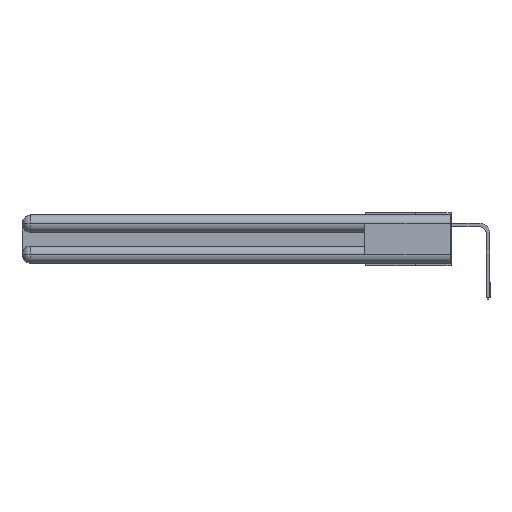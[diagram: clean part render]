
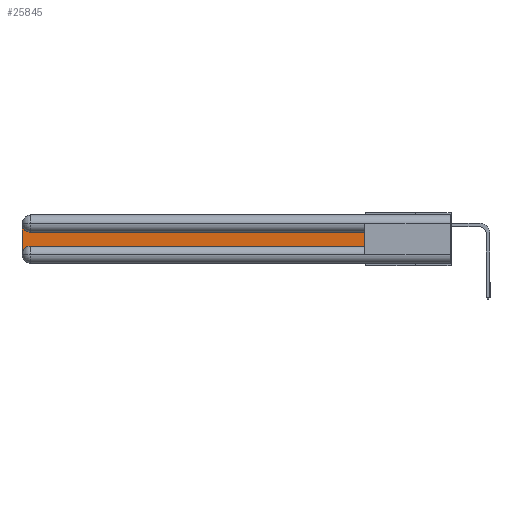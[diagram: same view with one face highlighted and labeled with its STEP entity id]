
A CAD part, left-side view. The second image highlights one B-rep face of the part: STEP entity #25845.
In plain terms, the highlighted planar face has unit normal (-1, 0, 0).
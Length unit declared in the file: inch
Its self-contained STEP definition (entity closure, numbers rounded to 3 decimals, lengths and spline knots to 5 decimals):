
#1119 = ORIENTED_EDGE ( 'NONE', *, *, #12127, .T. ) ;
#1807 = CARTESIAN_POINT ( 'NONE',  ( 0.075, 0.6, -0.1225 ) ) ;
#2072 = DIRECTION ( 'NONE',  ( 1., 0., 0. ) ) ;
#2469 = ORIENTED_EDGE ( 'NONE', *, *, #16069, .T. ) ;
#2662 = DIRECTION ( 'NONE',  ( 0., 0., 1. ) ) ;
#2831 = DIRECTION ( 'NONE',  ( 0., 1., 0. ) ) ;
#3142 = ORIENTED_EDGE ( 'NONE', *, *, #17017, .T. ) ;
#3325 = LINE ( 'NONE', #16458, #4412 ) ;
#3398 = VECTOR ( 'NONE', #2662, 39.37008 ) ;
#3775 = LINE ( 'NONE', #17286, #15225 ) ;
#3799 = EDGE_CURVE ( 'NONE', #9371, #26437, #3325, .T. ) ;
#4103 = VERTEX_POINT ( 'NONE', #1807 ) ;
#4412 = VECTOR ( 'NONE', #5385, 39.37008 ) ;
#5385 = DIRECTION ( 'NONE',  ( 0., -1., 0. ) ) ;
#5454 = AXIS2_PLACEMENT_3D ( 'NONE', #15026, #21813, #8323 ) ;
#5946 = FACE_OUTER_BOUND ( 'NONE', #22293, .T. ) ;
#6740 = CIRCLE ( 'NONE', #21140, 0.06 ) ;
#6820 = CARTESIAN_POINT ( 'NONE',  ( 0.075, 3., -0.1225 ) ) ;
#7042 = CARTESIAN_POINT ( 'NONE',  ( 0.075, 2.94, -0.2175 ) ) ;
#8323 = DIRECTION ( 'NONE',  ( 0., 0., -1. ) ) ;
#9371 = VERTEX_POINT ( 'NONE', #7042 ) ;
#10769 = VERTEX_POINT ( 'NONE', #17745 ) ;
#12127 = EDGE_CURVE ( 'NONE', #26437, #4103, #21660, .T. ) ;
#12393 = CIRCLE ( 'NONE', #5454, 0.06 ) ;
#13222 = EDGE_CURVE ( 'NONE', #4103, #14517, #17979, .T. ) ;
#13375 = CARTESIAN_POINT ( 'NONE',  ( 0.075, 0.6, -0.2175 ) ) ;
#14067 = VECTOR ( 'NONE', #2831, 39.37008 ) ;
#14517 = VERTEX_POINT ( 'NONE', #19823 ) ;
#15016 = ORIENTED_EDGE ( 'NONE', *, *, #17558, .T. ) ;
#15026 = CARTESIAN_POINT ( 'NONE',  ( 0.075, 2.94, -0.0625 ) ) ;
#15225 = VECTOR ( 'NONE', #28755, 39.37008 ) ;
#15980 = PLANE ( 'NONE',  #26422 ) ;
#16069 = EDGE_CURVE ( 'NONE', #10769, #9371, #6740, .T. ) ;
#16458 = CARTESIAN_POINT ( 'NONE',  ( 0.075, 0.6, -0.2175 ) ) ;
#17017 = EDGE_CURVE ( 'NONE', #25446, #10769, #3775, .T. ) ;
#17286 = CARTESIAN_POINT ( 'NONE',  ( 0.075, 3., -0.2175 ) ) ;
#17558 = EDGE_CURVE ( 'NONE', #14517, #25446, #12393, .T. ) ;
#17745 = CARTESIAN_POINT ( 'NONE',  ( 0.075, 3., -0.2775 ) ) ;
#17979 = LINE ( 'NONE', #29601, #14067 ) ;
#18504 = ORIENTED_EDGE ( 'NONE', *, *, #3799, .T. ) ;
#19823 = CARTESIAN_POINT ( 'NONE',  ( 0.075, 2.94, -0.1225 ) ) ;
#21140 = AXIS2_PLACEMENT_3D ( 'NONE', #23126, #23403, #25714 ) ;
#21191 = CARTESIAN_POINT ( 'NONE',  ( 0.075, 0.6, -0.2175 ) ) ;
#21319 = CARTESIAN_POINT ( 'NONE',  ( 0.075, 3., -0.0625 ) ) ;
#21660 = LINE ( 'NONE', #21191, #3398 ) ;
#21813 = DIRECTION ( 'NONE',  ( 1., 0., 0. ) ) ;
#22293 = EDGE_LOOP ( 'NONE', ( #22605, #15016, #3142, #2469, #18504, #1119 ) ) ;
#22605 = ORIENTED_EDGE ( 'NONE', *, *, #13222, .T. ) ;
#23126 = CARTESIAN_POINT ( 'NONE',  ( 0.075, 2.94, -0.2775 ) ) ;
#23403 = DIRECTION ( 'NONE',  ( 1., 0., 0. ) ) ;
#25081 = DIRECTION ( 'NONE',  ( 0., 0., -1. ) ) ;
#25446 = VERTEX_POINT ( 'NONE', #21319 ) ;
#25714 = DIRECTION ( 'NONE',  ( 0., 0., -1. ) ) ;
#25845 = ADVANCED_FACE ( 'NONE', ( #5946 ), #15980, .F. ) ;
#26422 = AXIS2_PLACEMENT_3D ( 'NONE', #6820, #2072, #25081 ) ;
#26437 = VERTEX_POINT ( 'NONE', #13375 ) ;
#28755 = DIRECTION ( 'NONE',  ( 0., 0., -1. ) ) ;
#29601 = CARTESIAN_POINT ( 'NONE',  ( 0.075, 0.6, -0.1225 ) ) ;
